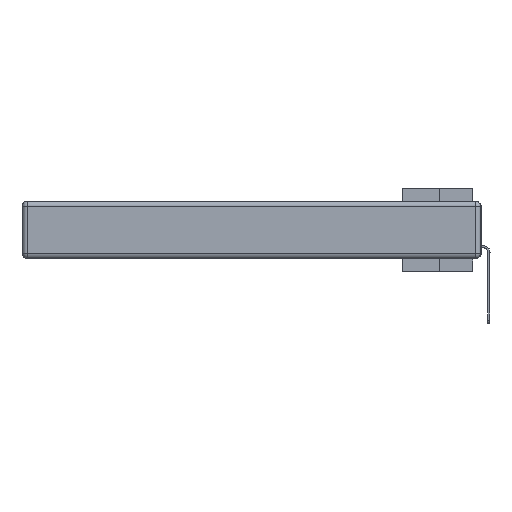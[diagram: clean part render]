
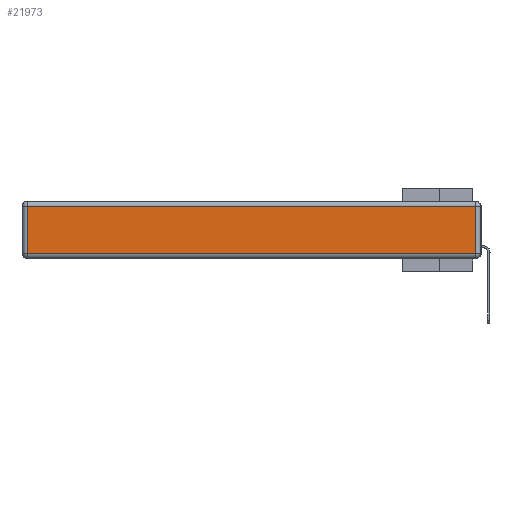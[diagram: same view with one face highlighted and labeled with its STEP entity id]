
A CAD part, left-side view. The second image highlights one B-rep face of the part: STEP entity #21973.
In plain terms, the highlighted planar face has unit normal (-1, 0, 0).
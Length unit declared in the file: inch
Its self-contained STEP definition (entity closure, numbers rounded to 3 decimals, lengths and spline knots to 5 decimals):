
#1014 = CARTESIAN_POINT ( 'NONE',  ( 0., 2.75, -0.03 ) ) ;
#1978 = CARTESIAN_POINT ( 'NONE',  ( 0., 0.03, -0.313 ) ) ;
#2230 = LINE ( 'NONE', #7874, #8444 ) ;
#2638 = VERTEX_POINT ( 'NONE', #36385 ) ;
#2859 = ORIENTED_EDGE ( 'NONE', *, *, #21793, .T. ) ;
#3453 = VERTEX_POINT ( 'NONE', #5715 ) ;
#4912 = ORIENTED_EDGE ( 'NONE', *, *, #25127, .T. ) ;
#5355 = CARTESIAN_POINT ( 'NONE',  ( 0., 2.72, -0.03 ) ) ;
#5715 = CARTESIAN_POINT ( 'NONE',  ( 0., 2.72, -0.313 ) ) ;
#7874 = CARTESIAN_POINT ( 'NONE',  ( 0., 0.03, -0.343 ) ) ;
#8444 = VECTOR ( 'NONE', #35750, 39.37008 ) ;
#9883 = EDGE_CURVE ( 'NONE', #11609, #2638, #2230, .T. ) ;
#10058 = VERTEX_POINT ( 'NONE', #5355 ) ;
#10549 = LINE ( 'NONE', #34196, #36706 ) ;
#11609 = VERTEX_POINT ( 'NONE', #1978 ) ;
#12333 = DIRECTION ( 'NONE',  ( 0., 1., 0. ) ) ;
#14332 = DIRECTION ( 'NONE',  ( 0., 0., -1. ) ) ;
#14673 = AXIS2_PLACEMENT_3D ( 'NONE', #20762, #14924, #34660 ) ;
#14924 = DIRECTION ( 'NONE',  ( -1., 0., 0. ) ) ;
#15428 = EDGE_LOOP ( 'NONE', ( #4912, #23520, #27409, #2859 ) ) ;
#16851 = EDGE_CURVE ( 'NONE', #2638, #10058, #35440, .T. ) ;
#17135 = LINE ( 'NONE', #34483, #22487 ) ;
#17772 = VECTOR ( 'NONE', #12333, 39.37008 ) ;
#19948 = FACE_OUTER_BOUND ( 'NONE', #15428, .T. ) ;
#20762 = CARTESIAN_POINT ( 'NONE',  ( 0., 0., -0.343 ) ) ;
#21793 = EDGE_CURVE ( 'NONE', #10058, #3453, #10549, .T. ) ;
#21973 = ADVANCED_FACE ( 'NONE', ( #19948 ), #26440, .T. ) ;
#22487 = VECTOR ( 'NONE', #26029, 39.37008 ) ;
#23520 = ORIENTED_EDGE ( 'NONE', *, *, #9883, .T. ) ;
#25127 = EDGE_CURVE ( 'NONE', #3453, #11609, #17135, .T. ) ;
#26029 = DIRECTION ( 'NONE',  ( 0., -1., 0. ) ) ;
#26440 = PLANE ( 'NONE',  #14673 ) ;
#27409 = ORIENTED_EDGE ( 'NONE', *, *, #16851, .T. ) ;
#34196 = CARTESIAN_POINT ( 'NONE',  ( 0., 2.72, -0.343 ) ) ;
#34483 = CARTESIAN_POINT ( 'NONE',  ( 0., 0., -0.313 ) ) ;
#34660 = DIRECTION ( 'NONE',  ( 0., 0., 1. ) ) ;
#35440 = LINE ( 'NONE', #1014, #17772 ) ;
#35750 = DIRECTION ( 'NONE',  ( 0., 0., 1. ) ) ;
#36385 = CARTESIAN_POINT ( 'NONE',  ( 0., 0.03, -0.03 ) ) ;
#36706 = VECTOR ( 'NONE', #14332, 39.37008 ) ;
